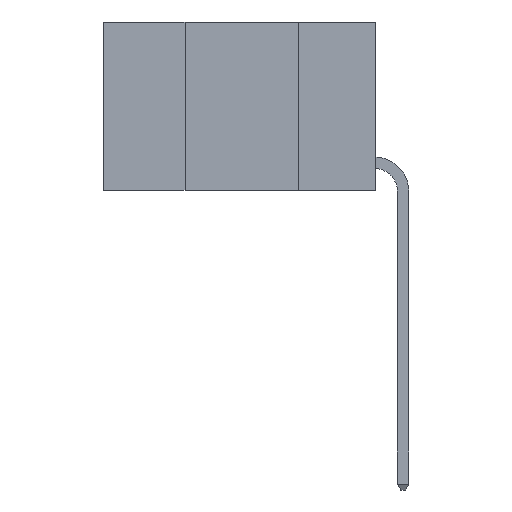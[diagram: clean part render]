
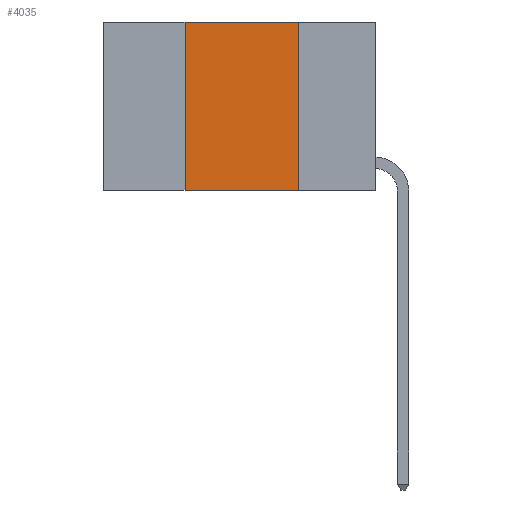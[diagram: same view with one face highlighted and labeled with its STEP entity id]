
A CAD part, left-side view. The second image highlights one B-rep face of the part: STEP entity #4035.
In plain terms, the highlighted planar face has unit normal (-1, 0, 0).
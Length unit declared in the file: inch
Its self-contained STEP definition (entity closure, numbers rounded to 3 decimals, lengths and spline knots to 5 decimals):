
#148 = VERTEX_POINT ( 'NONE', #1790 ) ;
#171 = DIRECTION ( 'NONE',  ( 0., 0., -1. ) ) ;
#613 = VECTOR ( 'NONE', #6154, 39.37008 ) ;
#792 = DIRECTION ( 'NONE',  ( 0., 0., 1. ) ) ;
#906 = EDGE_CURVE ( 'NONE', #9161, #10450, #8409, .T. ) ;
#1165 = AXIS2_PLACEMENT_3D ( 'NONE', #9942, #5251, #171 ) ;
#1198 = CARTESIAN_POINT ( 'NONE',  ( 0., 0.6, -0.37 ) ) ;
#1450 = EDGE_CURVE ( 'NONE', #10450, #148, #7935, .T. ) ;
#1735 = EDGE_CURVE ( 'NONE', #9161, #5171, #5116, .T. ) ;
#1790 = CARTESIAN_POINT ( 'NONE',  ( 0., 0.17, 0. ) ) ;
#2277 = ORIENTED_EDGE ( 'NONE', *, *, #3770, .F. ) ;
#2405 = ORIENTED_EDGE ( 'NONE', *, *, #1450, .F. ) ;
#2428 = ORIENTED_EDGE ( 'NONE', *, *, #906, .F. ) ;
#2439 = ORIENTED_EDGE ( 'NONE', *, *, #1735, .T. ) ;
#3119 = FACE_OUTER_BOUND ( 'NONE', #8614, .T. ) ;
#3770 = EDGE_CURVE ( 'NONE', #148, #5171, #4047, .T. ) ;
#4035 = ADVANCED_FACE ( 'NONE', ( #3119 ), #8369, .F. ) ;
#4047 = LINE ( 'NONE', #9585, #8014 ) ;
#4182 = CARTESIAN_POINT ( 'NONE',  ( 0., 0.6, 0. ) ) ;
#4371 = CARTESIAN_POINT ( 'NONE',  ( 0., 0.17, -0.37 ) ) ;
#5116 = LINE ( 'NONE', #1198, #613 ) ;
#5171 = VERTEX_POINT ( 'NONE', #4371 ) ;
#5251 = DIRECTION ( 'NONE',  ( 1., 0., 0. ) ) ;
#5794 = CARTESIAN_POINT ( 'NONE',  ( 0., 0.42, 0. ) ) ;
#6154 = DIRECTION ( 'NONE',  ( 0., -1., 0. ) ) ;
#7097 = CARTESIAN_POINT ( 'NONE',  ( 0., 0.42, -0.37 ) ) ;
#7251 = DIRECTION ( 'NONE',  ( 0., 0., -1. ) ) ;
#7548 = CARTESIAN_POINT ( 'NONE',  ( 0., 0.42, 0. ) ) ;
#7692 = VECTOR ( 'NONE', #9716, 39.37008 ) ;
#7935 = LINE ( 'NONE', #4182, #7692 ) ;
#8014 = VECTOR ( 'NONE', #7251, 39.37008 ) ;
#8369 = PLANE ( 'NONE',  #1165 ) ;
#8409 = LINE ( 'NONE', #5794, #8430 ) ;
#8430 = VECTOR ( 'NONE', #792, 39.37008 ) ;
#8614 = EDGE_LOOP ( 'NONE', ( #2277, #2405, #2428, #2439 ) ) ;
#9161 = VERTEX_POINT ( 'NONE', #7097 ) ;
#9585 = CARTESIAN_POINT ( 'NONE',  ( 0., 0.17, 0. ) ) ;
#9716 = DIRECTION ( 'NONE',  ( 0., -1., 0. ) ) ;
#9942 = CARTESIAN_POINT ( 'NONE',  ( 0., 0.6, 0. ) ) ;
#10450 = VERTEX_POINT ( 'NONE', #7548 ) ;
